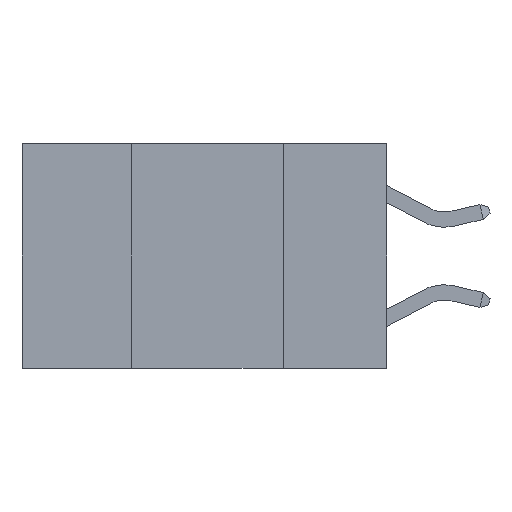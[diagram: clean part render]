
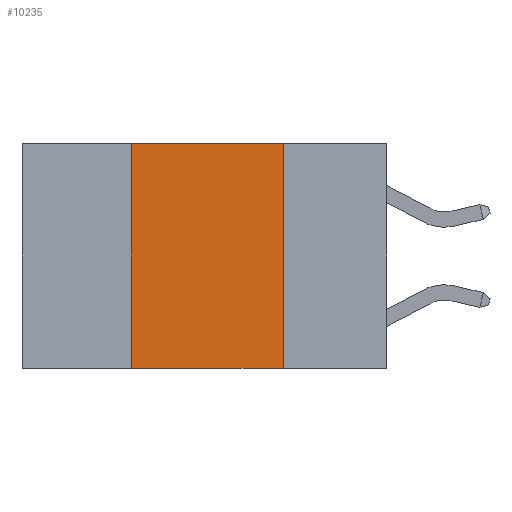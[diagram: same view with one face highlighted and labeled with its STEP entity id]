
A CAD part, left-side view. The second image highlights one B-rep face of the part: STEP entity #10235.
In plain terms, the highlighted planar face has unit normal (-1, 0, 0).
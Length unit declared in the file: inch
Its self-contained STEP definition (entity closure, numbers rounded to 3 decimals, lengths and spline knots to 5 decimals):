
#124 = ORIENTED_EDGE ( 'NONE', *, *, #682, .F. ) ;
#682 = EDGE_CURVE ( 'NONE', #10743, #6131, #2861, .T. ) ;
#801 = DIRECTION ( 'NONE',  ( 0., -1., 0. ) ) ;
#855 = EDGE_CURVE ( 'NONE', #6131, #5859, #1210, .T. ) ;
#897 = FACE_OUTER_BOUND ( 'NONE', #2739, .T. ) ;
#1210 = LINE ( 'NONE', #6330, #9729 ) ;
#1868 = CARTESIAN_POINT ( 'NONE',  ( 0., 0.42, 0. ) ) ;
#2204 = ORIENTED_EDGE ( 'NONE', *, *, #10469, .F. ) ;
#2536 = CARTESIAN_POINT ( 'NONE',  ( 0., 0.17, -0.37 ) ) ;
#2739 = EDGE_LOOP ( 'NONE', ( #3807, #124, #2204, #2807 ) ) ;
#2803 = LINE ( 'NONE', #1868, #9542 ) ;
#2807 = ORIENTED_EDGE ( 'NONE', *, *, #10869, .T. ) ;
#2861 = LINE ( 'NONE', #6972, #9591 ) ;
#3699 = DIRECTION ( 'NONE',  ( 0., 0., -1. ) ) ;
#3803 = LINE ( 'NONE', #9435, #8199 ) ;
#3807 = ORIENTED_EDGE ( 'NONE', *, *, #855, .F. ) ;
#4199 = CARTESIAN_POINT ( 'NONE',  ( 0., 0.6, 0. ) ) ;
#5084 = DIRECTION ( 'NONE',  ( 0., -1., 0. ) ) ;
#5569 = CARTESIAN_POINT ( 'NONE',  ( 0., 0.42, -0.37 ) ) ;
#5739 = AXIS2_PLACEMENT_3D ( 'NONE', #4199, #11190, #5978 ) ;
#5859 = VERTEX_POINT ( 'NONE', #2536 ) ;
#5978 = DIRECTION ( 'NONE',  ( 0., 0., -1. ) ) ;
#6131 = VERTEX_POINT ( 'NONE', #7364 ) ;
#6330 = CARTESIAN_POINT ( 'NONE',  ( 0., 0.17, 0. ) ) ;
#6335 = DIRECTION ( 'NONE',  ( 0., 0., 1. ) ) ;
#6968 = VERTEX_POINT ( 'NONE', #5569 ) ;
#6972 = CARTESIAN_POINT ( 'NONE',  ( 0., 0.6, 0. ) ) ;
#7364 = CARTESIAN_POINT ( 'NONE',  ( 0., 0.17, 0. ) ) ;
#8199 = VECTOR ( 'NONE', #5084, 39.37008 ) ;
#9435 = CARTESIAN_POINT ( 'NONE',  ( 0., 0.6, -0.37 ) ) ;
#9542 = VECTOR ( 'NONE', #6335, 39.37008 ) ;
#9591 = VECTOR ( 'NONE', #801, 39.37008 ) ;
#9729 = VECTOR ( 'NONE', #3699, 39.37008 ) ;
#10235 = ADVANCED_FACE ( 'NONE', ( #897 ), #10310, .F. ) ;
#10310 = PLANE ( 'NONE',  #5739 ) ;
#10469 = EDGE_CURVE ( 'NONE', #6968, #10743, #2803, .T. ) ;
#10743 = VERTEX_POINT ( 'NONE', #10991 ) ;
#10869 = EDGE_CURVE ( 'NONE', #6968, #5859, #3803, .T. ) ;
#10991 = CARTESIAN_POINT ( 'NONE',  ( 0., 0.42, 0. ) ) ;
#11190 = DIRECTION ( 'NONE',  ( 1., 0., 0. ) ) ;
